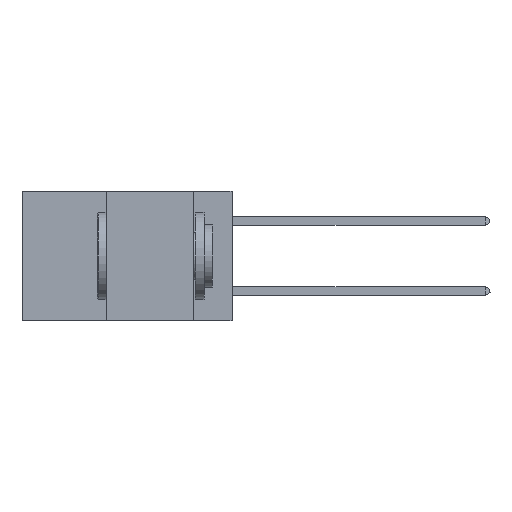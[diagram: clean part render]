
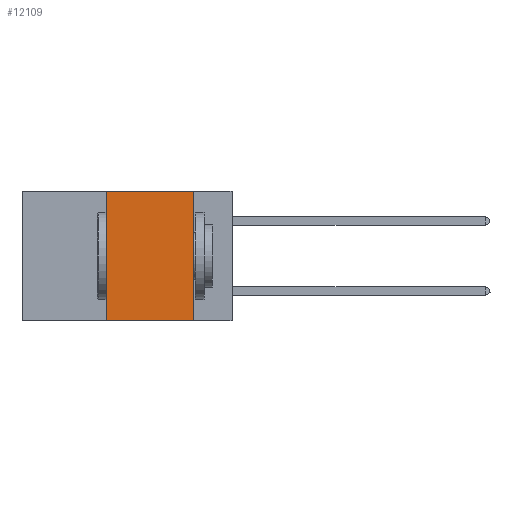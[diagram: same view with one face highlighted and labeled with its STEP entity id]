
A CAD part, left-side view. The second image highlights one B-rep face of the part: STEP entity #12109.
In plain terms, the highlighted planar face has unit normal (-1, 0, 0).
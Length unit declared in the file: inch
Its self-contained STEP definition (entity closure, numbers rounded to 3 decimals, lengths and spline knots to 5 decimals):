
#748 = PLANE ( 'NONE',  #11367 ) ;
#920 = EDGE_CURVE ( 'NONE', #1452, #23605, #1430, .T. ) ;
#1430 = LINE ( 'NONE', #3397, #18575 ) ;
#1452 = VERTEX_POINT ( 'NONE', #16953 ) ;
#1916 = LINE ( 'NONE', #9362, #22902 ) ;
#2863 = DIRECTION ( 'NONE',  ( 1., 0., 0. ) ) ;
#3010 = CARTESIAN_POINT ( 'NONE',  ( 0., 0.11, 0. ) ) ;
#3397 = CARTESIAN_POINT ( 'NONE',  ( 0., 0.36, 0. ) ) ;
#4176 = CARTESIAN_POINT ( 'NONE',  ( 0., 0.11, 0. ) ) ;
#4519 = CARTESIAN_POINT ( 'NONE',  ( 0., 0.11, -0.37 ) ) ;
#4553 = CARTESIAN_POINT ( 'NONE',  ( 0., 0.6, -0.37 ) ) ;
#5096 = DIRECTION ( 'NONE',  ( 0., 0., 1. ) ) ;
#5218 = VERTEX_POINT ( 'NONE', #3010 ) ;
#5631 = ORIENTED_EDGE ( 'NONE', *, *, #25766, .T. ) ;
#8567 = DIRECTION ( 'NONE',  ( 0., -1., 0. ) ) ;
#9180 = DIRECTION ( 'NONE',  ( 0., -1., 0. ) ) ;
#9362 = CARTESIAN_POINT ( 'NONE',  ( 0., 0.6, 0. ) ) ;
#11367 = AXIS2_PLACEMENT_3D ( 'NONE', #14986, #2863, #19134 ) ;
#11398 = EDGE_CURVE ( 'NONE', #5218, #24300, #11450, .T. ) ;
#11450 = LINE ( 'NONE', #4176, #21603 ) ;
#12109 = ADVANCED_FACE ( 'NONE', ( #14974 ), #748, .F. ) ;
#13287 = ORIENTED_EDGE ( 'NONE', *, *, #11398, .F. ) ;
#14974 = FACE_OUTER_BOUND ( 'NONE', #20670, .T. ) ;
#14986 = CARTESIAN_POINT ( 'NONE',  ( 0., 0.6, 0. ) ) ;
#16953 = CARTESIAN_POINT ( 'NONE',  ( 0., 0.36, -0.37 ) ) ;
#18098 = VECTOR ( 'NONE', #8567, 39.37008 ) ;
#18575 = VECTOR ( 'NONE', #5096, 39.37008 ) ;
#18758 = CARTESIAN_POINT ( 'NONE',  ( 0., 0.36, 0. ) ) ;
#19134 = DIRECTION ( 'NONE',  ( 0., 0., -1. ) ) ;
#20670 = EDGE_LOOP ( 'NONE', ( #13287, #25206, #21031, #5631 ) ) ;
#21031 = ORIENTED_EDGE ( 'NONE', *, *, #920, .F. ) ;
#21603 = VECTOR ( 'NONE', #22408, 39.37008 ) ;
#22240 = LINE ( 'NONE', #4553, #18098 ) ;
#22408 = DIRECTION ( 'NONE',  ( 0., 0., -1. ) ) ;
#22902 = VECTOR ( 'NONE', #9180, 39.37008 ) ;
#23605 = VERTEX_POINT ( 'NONE', #18758 ) ;
#24300 = VERTEX_POINT ( 'NONE', #4519 ) ;
#25205 = EDGE_CURVE ( 'NONE', #23605, #5218, #1916, .T. ) ;
#25206 = ORIENTED_EDGE ( 'NONE', *, *, #25205, .F. ) ;
#25766 = EDGE_CURVE ( 'NONE', #1452, #24300, #22240, .T. ) ;
